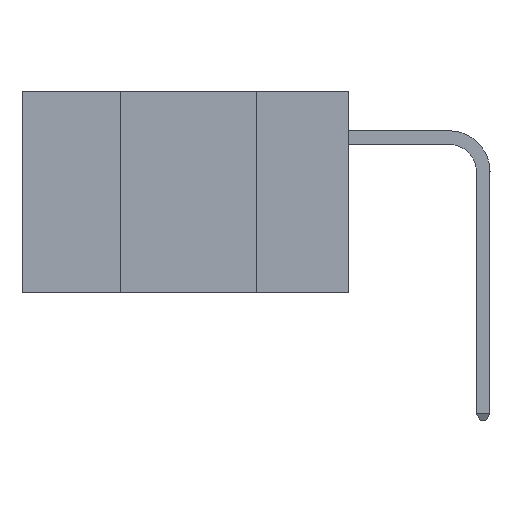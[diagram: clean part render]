
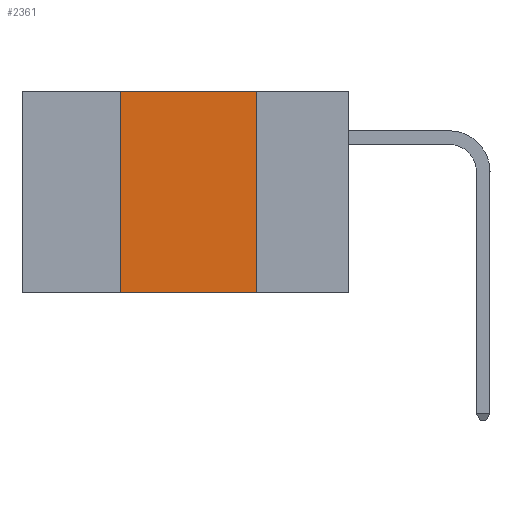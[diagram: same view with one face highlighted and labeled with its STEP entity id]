
A CAD part, left-side view. The second image highlights one B-rep face of the part: STEP entity #2361.
In plain terms, the highlighted planar face has unit normal (-1, 0, 0).
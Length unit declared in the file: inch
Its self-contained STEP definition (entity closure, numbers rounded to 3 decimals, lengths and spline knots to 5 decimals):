
#239 = CARTESIAN_POINT ( 'NONE',  ( 0., 0.17, -0.37 ) ) ;
#457 = EDGE_CURVE ( 'NONE', #8580, #3533, #1059, .T. ) ;
#906 = DIRECTION ( 'NONE',  ( 1., 0., 0. ) ) ;
#1059 = LINE ( 'NONE', #1533, #3322 ) ;
#1533 = CARTESIAN_POINT ( 'NONE',  ( 0., 0.17, 0. ) ) ;
#2361 = ADVANCED_FACE ( 'NONE', ( #13216 ), #4142, .F. ) ;
#3322 = VECTOR ( 'NONE', #11966, 39.37008 ) ;
#3522 = EDGE_CURVE ( 'NONE', #5180, #6798, #7207, .T. ) ;
#3533 = VERTEX_POINT ( 'NONE', #239 ) ;
#3774 = VECTOR ( 'NONE', #11601, 39.37008 ) ;
#4142 = PLANE ( 'NONE',  #9467 ) ;
#5180 = VERTEX_POINT ( 'NONE', #12795 ) ;
#5338 = CARTESIAN_POINT ( 'NONE',  ( 0., 0.42, 0. ) ) ;
#6245 = CARTESIAN_POINT ( 'NONE',  ( 0., 0.6, 0. ) ) ;
#6340 = EDGE_CURVE ( 'NONE', #5180, #3533, #7316, .T. ) ;
#6401 = DIRECTION ( 'NONE',  ( 0., 0., 1. ) ) ;
#6798 = VERTEX_POINT ( 'NONE', #5338 ) ;
#7207 = LINE ( 'NONE', #8500, #8969 ) ;
#7316 = LINE ( 'NONE', #10571, #3774 ) ;
#7336 = ORIENTED_EDGE ( 'NONE', *, *, #3522, .F. ) ;
#7896 = ORIENTED_EDGE ( 'NONE', *, *, #10584, .F. ) ;
#8192 = ORIENTED_EDGE ( 'NONE', *, *, #457, .F. ) ;
#8500 = CARTESIAN_POINT ( 'NONE',  ( 0., 0.42, 0. ) ) ;
#8529 = LINE ( 'NONE', #6245, #12837 ) ;
#8580 = VERTEX_POINT ( 'NONE', #9251 ) ;
#8969 = VECTOR ( 'NONE', #6401, 39.37008 ) ;
#9251 = CARTESIAN_POINT ( 'NONE',  ( 0., 0.17, 0. ) ) ;
#9467 = AXIS2_PLACEMENT_3D ( 'NONE', #11214, #906, #11301 ) ;
#10571 = CARTESIAN_POINT ( 'NONE',  ( 0., 0.6, -0.37 ) ) ;
#10584 = EDGE_CURVE ( 'NONE', #6798, #8580, #8529, .T. ) ;
#11061 = ORIENTED_EDGE ( 'NONE', *, *, #6340, .T. ) ;
#11214 = CARTESIAN_POINT ( 'NONE',  ( 0., 0.6, 0. ) ) ;
#11301 = DIRECTION ( 'NONE',  ( 0., 0., -1. ) ) ;
#11319 = DIRECTION ( 'NONE',  ( 0., -1., 0. ) ) ;
#11530 = EDGE_LOOP ( 'NONE', ( #8192, #7896, #7336, #11061 ) ) ;
#11601 = DIRECTION ( 'NONE',  ( 0., -1., 0. ) ) ;
#11966 = DIRECTION ( 'NONE',  ( 0., 0., -1. ) ) ;
#12795 = CARTESIAN_POINT ( 'NONE',  ( 0., 0.42, -0.37 ) ) ;
#12837 = VECTOR ( 'NONE', #11319, 39.37008 ) ;
#13216 = FACE_OUTER_BOUND ( 'NONE', #11530, .T. ) ;
